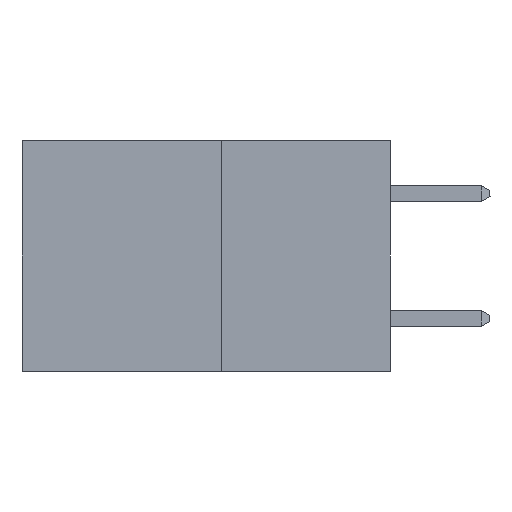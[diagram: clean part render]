
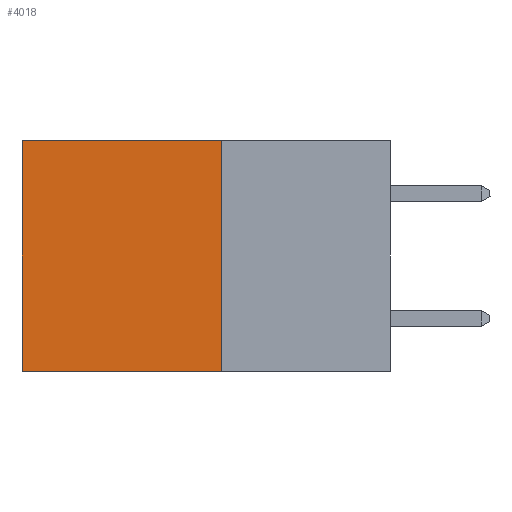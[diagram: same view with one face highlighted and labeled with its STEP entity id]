
A CAD part, left-side view. The second image highlights one B-rep face of the part: STEP entity #4018.
In plain terms, the highlighted planar face has unit normal (-1, 0, 0).
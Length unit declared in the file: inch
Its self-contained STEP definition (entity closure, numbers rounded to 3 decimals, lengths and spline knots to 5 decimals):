
#459 = VERTEX_POINT ( 'NONE', #15830 ) ;
#1231 = VERTEX_POINT ( 'NONE', #5002 ) ;
#2236 = VECTOR ( 'NONE', #10672, 39.37008 ) ;
#2992 = ORIENTED_EDGE ( 'NONE', *, *, #3594, .F. ) ;
#3122 = CARTESIAN_POINT ( 'NONE',  ( 0.277, 0.27, 0. ) ) ;
#3594 = EDGE_CURVE ( 'NONE', #16248, #1231, #6391, .T. ) ;
#3871 = ORIENTED_EDGE ( 'NONE', *, *, #11901, .F. ) ;
#4018 = ADVANCED_FACE ( 'NONE', ( #7157 ), #4486, .F. ) ;
#4296 = DIRECTION ( 'NONE',  ( 0., 0., -1. ) ) ;
#4415 = DIRECTION ( 'NONE',  ( 1., 0., 0. ) ) ;
#4486 = PLANE ( 'NONE',  #5829 ) ;
#4568 = EDGE_CURVE ( 'NONE', #459, #1231, #15531, .T. ) ;
#4729 = CARTESIAN_POINT ( 'NONE',  ( 0.277, 0.27, -0.37 ) ) ;
#4748 = CARTESIAN_POINT ( 'NONE',  ( 0.277, 0.27, -0.37 ) ) ;
#5002 = CARTESIAN_POINT ( 'NONE',  ( 0.277, 0.59, -0.37 ) ) ;
#5829 = AXIS2_PLACEMENT_3D ( 'NONE', #4729, #4415, #4296 ) ;
#6174 = LINE ( 'NONE', #12042, #12395 ) ;
#6263 = DIRECTION ( 'NONE',  ( 0., 0., -1. ) ) ;
#6391 = LINE ( 'NONE', #13061, #15953 ) ;
#6434 = LINE ( 'NONE', #4748, #12637 ) ;
#7157 = FACE_OUTER_BOUND ( 'NONE', #7437, .T. ) ;
#7437 = EDGE_LOOP ( 'NONE', ( #10733, #2992, #3871, #15890 ) ) ;
#8669 = CARTESIAN_POINT ( 'NONE',  ( 0.277, 0.27, -0.37 ) ) ;
#9023 = VERTEX_POINT ( 'NONE', #3122 ) ;
#10672 = DIRECTION ( 'NONE',  ( 0., 0., -1. ) ) ;
#10733 = ORIENTED_EDGE ( 'NONE', *, *, #4568, .T. ) ;
#10738 = CARTESIAN_POINT ( 'NONE',  ( 0.277, 0.59, -0.37 ) ) ;
#11901 = EDGE_CURVE ( 'NONE', #9023, #16248, #6434, .T. ) ;
#12042 = CARTESIAN_POINT ( 'NONE',  ( 0.277, 0.27, 0. ) ) ;
#12096 = DIRECTION ( 'NONE',  ( 0., 1., 0. ) ) ;
#12395 = VECTOR ( 'NONE', #12096, 39.37008 ) ;
#12637 = VECTOR ( 'NONE', #6263, 39.37008 ) ;
#13061 = CARTESIAN_POINT ( 'NONE',  ( 0.277, 0.27, -0.37 ) ) ;
#13095 = EDGE_CURVE ( 'NONE', #9023, #459, #6174, .T. ) ;
#13921 = DIRECTION ( 'NONE',  ( 0., 1., 0. ) ) ;
#15531 = LINE ( 'NONE', #10738, #2236 ) ;
#15830 = CARTESIAN_POINT ( 'NONE',  ( 0.277, 0.59, 0. ) ) ;
#15890 = ORIENTED_EDGE ( 'NONE', *, *, #13095, .T. ) ;
#15953 = VECTOR ( 'NONE', #13921, 39.37008 ) ;
#16248 = VERTEX_POINT ( 'NONE', #8669 ) ;
